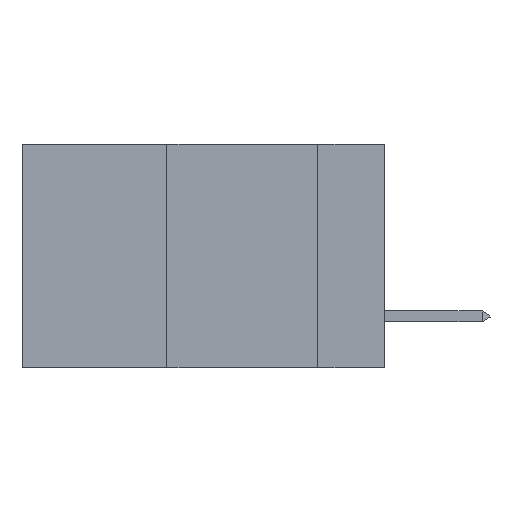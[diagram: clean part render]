
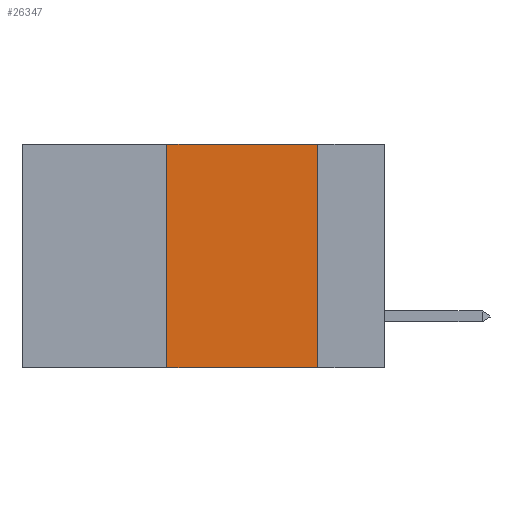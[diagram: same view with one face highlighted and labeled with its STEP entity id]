
A CAD part, left-side view. The second image highlights one B-rep face of the part: STEP entity #26347.
In plain terms, the highlighted planar face has unit normal (-1, 0, 0).
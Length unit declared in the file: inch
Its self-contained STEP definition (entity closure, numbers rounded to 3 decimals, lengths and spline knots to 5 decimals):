
#382 = VERTEX_POINT ( 'NONE', #17812 ) ;
#759 = VERTEX_POINT ( 'NONE', #10921 ) ;
#1488 = ORIENTED_EDGE ( 'NONE', *, *, #21443, .F. ) ;
#2722 = VECTOR ( 'NONE', #19212, 39.37008 ) ;
#2796 = CARTESIAN_POINT ( 'NONE',  ( 0., 0.11, -0.37 ) ) ;
#3653 = VECTOR ( 'NONE', #10927, 39.37008 ) ;
#3805 = VECTOR ( 'NONE', #14556, 39.37008 ) ;
#4219 = CARTESIAN_POINT ( 'NONE',  ( 0., 0.6, 0. ) ) ;
#6964 = VECTOR ( 'NONE', #24818, 39.37008 ) ;
#7016 = CARTESIAN_POINT ( 'NONE',  ( 0., 0.36, 0. ) ) ;
#7360 = CARTESIAN_POINT ( 'NONE',  ( 0., 0.11, 0. ) ) ;
#7496 = DIRECTION ( 'NONE',  ( 1., 0., 0. ) ) ;
#8323 = VERTEX_POINT ( 'NONE', #2796 ) ;
#9134 = EDGE_LOOP ( 'NONE', ( #1488, #23917, #20765, #22933 ) ) ;
#9175 = LINE ( 'NONE', #7016, #3653 ) ;
#9212 = FACE_OUTER_BOUND ( 'NONE', #9134, .T. ) ;
#9891 = VERTEX_POINT ( 'NONE', #7360 ) ;
#9997 = EDGE_CURVE ( 'NONE', #382, #9891, #13792, .T. ) ;
#10921 = CARTESIAN_POINT ( 'NONE',  ( 0., 0.36, -0.37 ) ) ;
#10927 = DIRECTION ( 'NONE',  ( 0., 0., 1. ) ) ;
#11954 = AXIS2_PLACEMENT_3D ( 'NONE', #21719, #7496, #22073 ) ;
#13792 = LINE ( 'NONE', #4219, #6964 ) ;
#14556 = DIRECTION ( 'NONE',  ( 0., -1., 0. ) ) ;
#15048 = LINE ( 'NONE', #23285, #2722 ) ;
#15715 = PLANE ( 'NONE',  #11954 ) ;
#16128 = LINE ( 'NONE', #20609, #3805 ) ;
#16203 = EDGE_CURVE ( 'NONE', #759, #382, #9175, .T. ) ;
#17812 = CARTESIAN_POINT ( 'NONE',  ( 0., 0.36, 0. ) ) ;
#19212 = DIRECTION ( 'NONE',  ( 0., 0., -1. ) ) ;
#20609 = CARTESIAN_POINT ( 'NONE',  ( 0., 0.6, -0.37 ) ) ;
#20765 = ORIENTED_EDGE ( 'NONE', *, *, #16203, .F. ) ;
#21443 = EDGE_CURVE ( 'NONE', #9891, #8323, #15048, .T. ) ;
#21719 = CARTESIAN_POINT ( 'NONE',  ( 0., 0.6, 0. ) ) ;
#22073 = DIRECTION ( 'NONE',  ( 0., 0., -1. ) ) ;
#22933 = ORIENTED_EDGE ( 'NONE', *, *, #23995, .T. ) ;
#23285 = CARTESIAN_POINT ( 'NONE',  ( 0., 0.11, 0. ) ) ;
#23917 = ORIENTED_EDGE ( 'NONE', *, *, #9997, .F. ) ;
#23995 = EDGE_CURVE ( 'NONE', #759, #8323, #16128, .T. ) ;
#24818 = DIRECTION ( 'NONE',  ( 0., -1., 0. ) ) ;
#26347 = ADVANCED_FACE ( 'NONE', ( #9212 ), #15715, .F. ) ;
